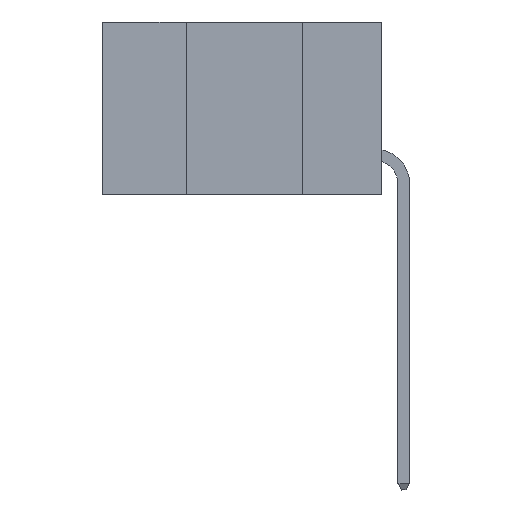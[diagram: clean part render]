
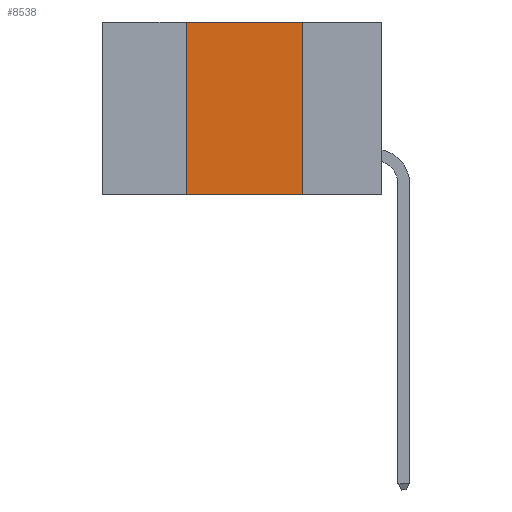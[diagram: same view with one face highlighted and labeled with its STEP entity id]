
A CAD part, left-side view. The second image highlights one B-rep face of the part: STEP entity #8538.
In plain terms, the highlighted planar face has unit normal (-1, 0, 0).
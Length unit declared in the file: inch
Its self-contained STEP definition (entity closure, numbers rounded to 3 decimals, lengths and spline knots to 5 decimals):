
#36 = EDGE_CURVE ( 'NONE', #1661, #19795, #16323, .T. ) ;
#934 = ORIENTED_EDGE ( 'NONE', *, *, #12784, .F. ) ;
#1367 = ORIENTED_EDGE ( 'NONE', *, *, #14084, .F. ) ;
#1661 = VERTEX_POINT ( 'NONE', #10793 ) ;
#2491 = CARTESIAN_POINT ( 'NONE',  ( 0., 0.42, 0. ) ) ;
#2777 = CARTESIAN_POINT ( 'NONE',  ( 0., 0.6, 0. ) ) ;
#3304 = EDGE_LOOP ( 'NONE', ( #1367, #19107, #934, #12169 ) ) ;
#3410 = VECTOR ( 'NONE', #7580, 39.37008 ) ;
#4282 = FACE_OUTER_BOUND ( 'NONE', #3304, .T. ) ;
#5193 = AXIS2_PLACEMENT_3D ( 'NONE', #9327, #11841, #8272 ) ;
#6344 = VERTEX_POINT ( 'NONE', #6666 ) ;
#6666 = CARTESIAN_POINT ( 'NONE',  ( 0., 0.17, 0. ) ) ;
#7093 = CARTESIAN_POINT ( 'NONE',  ( 0., 0.17, -0.37 ) ) ;
#7580 = DIRECTION ( 'NONE',  ( 0., -1., 0. ) ) ;
#7921 = VECTOR ( 'NONE', #10035, 39.37008 ) ;
#7923 = DIRECTION ( 'NONE',  ( 0., -1., 0. ) ) ;
#8033 = CARTESIAN_POINT ( 'NONE',  ( 0., 0.42, 0. ) ) ;
#8272 = DIRECTION ( 'NONE',  ( 0., 0., -1. ) ) ;
#8538 = ADVANCED_FACE ( 'NONE', ( #4282 ), #19824, .F. ) ;
#9327 = CARTESIAN_POINT ( 'NONE',  ( 0., 0.6, 0. ) ) ;
#10035 = DIRECTION ( 'NONE',  ( 0., 0., -1. ) ) ;
#10310 = EDGE_CURVE ( 'NONE', #15039, #6344, #17062, .T. ) ;
#10330 = LINE ( 'NONE', #2491, #16462 ) ;
#10793 = CARTESIAN_POINT ( 'NONE',  ( 0., 0.42, -0.37 ) ) ;
#11841 = DIRECTION ( 'NONE',  ( 1., 0., 0. ) ) ;
#11964 = VECTOR ( 'NONE', #7923, 39.37008 ) ;
#12169 = ORIENTED_EDGE ( 'NONE', *, *, #36, .T. ) ;
#12784 = EDGE_CURVE ( 'NONE', #1661, #15039, #10330, .T. ) ;
#14084 = EDGE_CURVE ( 'NONE', #6344, #19795, #21009, .T. ) ;
#14548 = CARTESIAN_POINT ( 'NONE',  ( 0., 0.6, -0.37 ) ) ;
#15039 = VERTEX_POINT ( 'NONE', #8033 ) ;
#16323 = LINE ( 'NONE', #14548, #11964 ) ;
#16462 = VECTOR ( 'NONE', #19037, 39.37008 ) ;
#16727 = CARTESIAN_POINT ( 'NONE',  ( 0., 0.17, 0. ) ) ;
#17062 = LINE ( 'NONE', #2777, #3410 ) ;
#19037 = DIRECTION ( 'NONE',  ( 0., 0., 1. ) ) ;
#19107 = ORIENTED_EDGE ( 'NONE', *, *, #10310, .F. ) ;
#19795 = VERTEX_POINT ( 'NONE', #7093 ) ;
#19824 = PLANE ( 'NONE',  #5193 ) ;
#21009 = LINE ( 'NONE', #16727, #7921 ) ;
